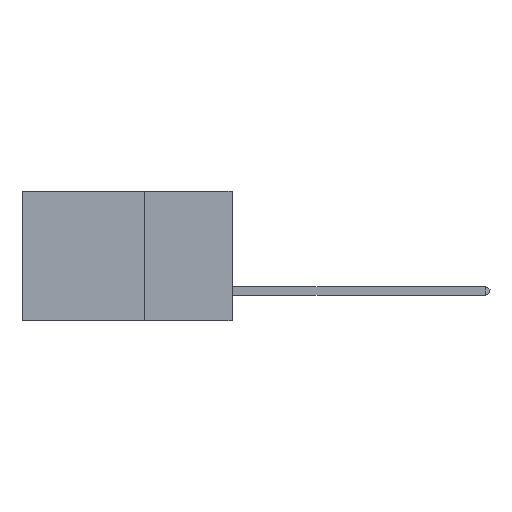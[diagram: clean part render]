
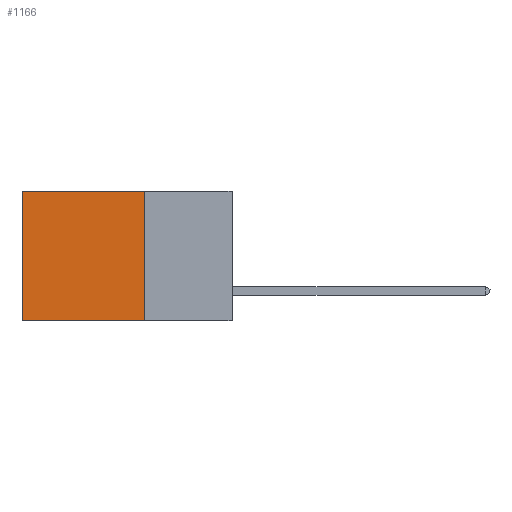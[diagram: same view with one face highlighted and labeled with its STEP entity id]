
A CAD part, left-side view. The second image highlights one B-rep face of the part: STEP entity #1166.
In plain terms, the highlighted planar face has unit normal (-1, 0, 0).
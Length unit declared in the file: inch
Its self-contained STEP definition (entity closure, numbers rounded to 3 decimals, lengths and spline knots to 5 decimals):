
#256 = VERTEX_POINT ( 'NONE', #12379 ) ;
#528 = VECTOR ( 'NONE', #14070, 39.37008 ) ;
#1166 = ADVANCED_FACE ( 'NONE', ( #14960 ), #15652, .F. ) ;
#1517 = CARTESIAN_POINT ( 'NONE',  ( 0.2875, 0.25, 0. ) ) ;
#3184 = DIRECTION ( 'NONE',  ( 0., 0., -1. ) ) ;
#4120 = VECTOR ( 'NONE', #11391, 39.37008 ) ;
#4325 = DIRECTION ( 'NONE',  ( 1., 0., 0. ) ) ;
#4417 = CARTESIAN_POINT ( 'NONE',  ( 0.2875, 0.6, 0. ) ) ;
#4617 = CARTESIAN_POINT ( 'NONE',  ( 0.2875, 0.6, 0. ) ) ;
#6326 = EDGE_CURVE ( 'NONE', #256, #13340, #8819, .T. ) ;
#6644 = VECTOR ( 'NONE', #7733, 39.37008 ) ;
#6755 = LINE ( 'NONE', #15221, #528 ) ;
#7733 = DIRECTION ( 'NONE',  ( 0., 1., 0. ) ) ;
#7819 = AXIS2_PLACEMENT_3D ( 'NONE', #10716, #4325, #3184 ) ;
#7834 = EDGE_CURVE ( 'NONE', #13340, #8859, #13813, .T. ) ;
#8443 = ORIENTED_EDGE ( 'NONE', *, *, #6326, .T. ) ;
#8819 = LINE ( 'NONE', #1517, #4120 ) ;
#8859 = VERTEX_POINT ( 'NONE', #12687 ) ;
#9699 = VERTEX_POINT ( 'NONE', #12343 ) ;
#10185 = ORIENTED_EDGE ( 'NONE', *, *, #14475, .F. ) ;
#10716 = CARTESIAN_POINT ( 'NONE',  ( 0.2875, 0.25, 0. ) ) ;
#10944 = EDGE_CURVE ( 'NONE', #256, #9699, #6755, .T. ) ;
#11391 = DIRECTION ( 'NONE',  ( 0., 1., 0. ) ) ;
#11473 = CARTESIAN_POINT ( 'NONE',  ( 0.2875, 0.25, -0.37 ) ) ;
#12265 = VECTOR ( 'NONE', #14288, 39.37008 ) ;
#12343 = CARTESIAN_POINT ( 'NONE',  ( 0.2875, 0.25, -0.37 ) ) ;
#12379 = CARTESIAN_POINT ( 'NONE',  ( 0.2875, 0.25, 0. ) ) ;
#12687 = CARTESIAN_POINT ( 'NONE',  ( 0.2875, 0.6, -0.37 ) ) ;
#12774 = ORIENTED_EDGE ( 'NONE', *, *, #10944, .F. ) ;
#13340 = VERTEX_POINT ( 'NONE', #4617 ) ;
#13813 = LINE ( 'NONE', #4417, #12265 ) ;
#14070 = DIRECTION ( 'NONE',  ( 0., 0., -1. ) ) ;
#14288 = DIRECTION ( 'NONE',  ( 0., 0., -1. ) ) ;
#14475 = EDGE_CURVE ( 'NONE', #9699, #8859, #15607, .T. ) ;
#14498 = ORIENTED_EDGE ( 'NONE', *, *, #7834, .T. ) ;
#14960 = FACE_OUTER_BOUND ( 'NONE', #15892, .T. ) ;
#15221 = CARTESIAN_POINT ( 'NONE',  ( 0.2875, 0.25, 0. ) ) ;
#15607 = LINE ( 'NONE', #11473, #6644 ) ;
#15652 = PLANE ( 'NONE',  #7819 ) ;
#15892 = EDGE_LOOP ( 'NONE', ( #14498, #10185, #12774, #8443 ) ) ;
